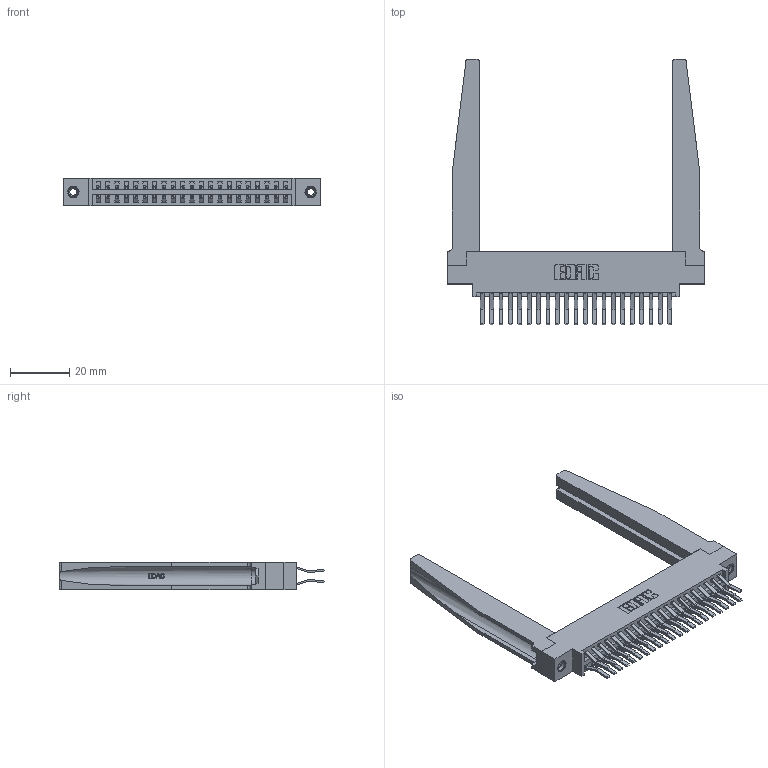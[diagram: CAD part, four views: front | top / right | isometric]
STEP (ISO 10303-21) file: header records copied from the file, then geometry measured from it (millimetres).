
FILE_DESCRIPTION (( 'STEP AP203' ), '1' );
FILE_NAME ('346-042-560-878.STEP', '2022-05-20T05:56:36', ( '' ), ( '' ), 'SwSTEP 2.0', 'SolidWorks 2020', '' );
FILE_SCHEMA (( 'CONFIG_CONTROL_DESIGN' ));
Length unit declared in the file: inch
Products named in the file (5): 345-250-001_345-250-001-102; 345-292-001_560 Tail; 346-220-078_345-220-078; 346 Part_0.170 Offset - 0.156 Dia-TH; 346-042-560-878
Assembly tree (47 placements, depth 2):
  346-042-560-878
    346 Part_0.170 Offset - 0.156 Dia-TH
    345-292-001_560 Tail  x42
    346-220-078_345-220-078  x2
    345-250-001_345-250-001-102  x2
Bounding box: 87.25 x 90.05 x 9.4 mm (x, y, z)
Volume: 15356.2 mm3; surface area: 18767.5 mm2
Topology: 47 solids, 47 shells, 2642 faces, 7747 edges, 5098 vertices
Faces by surface type: plane 1706, cylinder 884, bspline 36, cone 12, torus 4
Entity records: 21916 total; most frequent: CARTESIAN_POINT 4585, ORIENTED_EDGE 3406, DIRECTION 3081, EDGE_CURVE 1703, VECTOR 1389, LINE 1389, VERTEX_POINT 1128, AXIS2_PLACEMENT_3D 846
